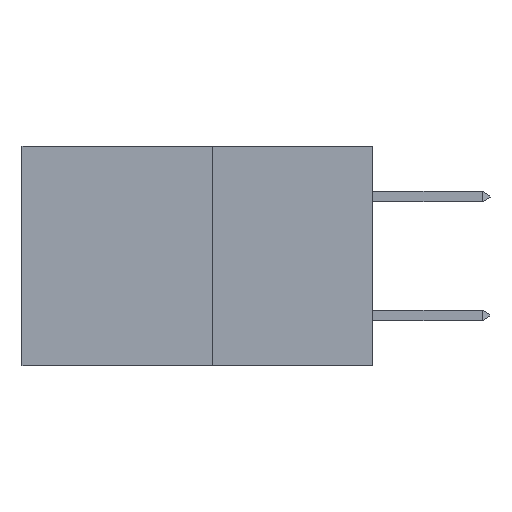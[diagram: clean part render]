
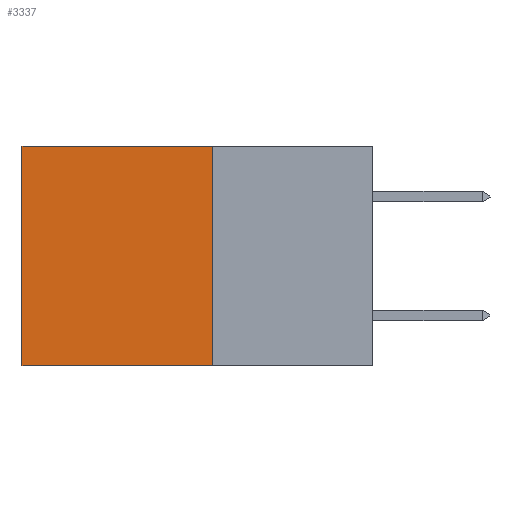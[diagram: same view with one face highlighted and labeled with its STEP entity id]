
A CAD part, left-side view. The second image highlights one B-rep face of the part: STEP entity #3337.
In plain terms, the highlighted planar face has unit normal (-1, 0, 0).
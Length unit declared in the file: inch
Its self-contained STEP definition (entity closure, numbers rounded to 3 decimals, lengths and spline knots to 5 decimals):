
#795 = DIRECTION ( 'NONE',  ( 0., 1., 0. ) ) ;
#839 = CARTESIAN_POINT ( 'NONE',  ( 0.277, 0.27, -0.37 ) ) ;
#1042 = VERTEX_POINT ( 'NONE', #9875 ) ;
#1061 = ORIENTED_EDGE ( 'NONE', *, *, #6107, .T. ) ;
#1336 = EDGE_CURVE ( 'NONE', #9723, #1696, #6829, .T. ) ;
#1437 = ORIENTED_EDGE ( 'NONE', *, *, #1336, .F. ) ;
#1644 = DIRECTION ( 'NONE',  ( 0., 1., 0. ) ) ;
#1651 = EDGE_CURVE ( 'NONE', #9723, #1042, #3816, .T. ) ;
#1696 = VERTEX_POINT ( 'NONE', #1767 ) ;
#1767 = CARTESIAN_POINT ( 'NONE',  ( 0.277, 0.27, -0.37 ) ) ;
#2977 = VECTOR ( 'NONE', #11805, 39.37008 ) ;
#3291 = CARTESIAN_POINT ( 'NONE',  ( 0.277, 0.59, -0.37 ) ) ;
#3337 = ADVANCED_FACE ( 'NONE', ( #3777 ), #9897, .F. ) ;
#3438 = EDGE_CURVE ( 'NONE', #1696, #5082, #12374, .T. ) ;
#3777 = FACE_OUTER_BOUND ( 'NONE', #3894, .T. ) ;
#3816 = LINE ( 'NONE', #8935, #8815 ) ;
#3894 = EDGE_LOOP ( 'NONE', ( #1061, #6743, #1437, #8344 ) ) ;
#5082 = VERTEX_POINT ( 'NONE', #3291 ) ;
#5830 = LINE ( 'NONE', #10865, #2977 ) ;
#6107 = EDGE_CURVE ( 'NONE', #1042, #5082, #5830, .T. ) ;
#6743 = ORIENTED_EDGE ( 'NONE', *, *, #3438, .F. ) ;
#6829 = LINE ( 'NONE', #10586, #9134 ) ;
#7911 = CARTESIAN_POINT ( 'NONE',  ( 0.277, 0.27, 0. ) ) ;
#8344 = ORIENTED_EDGE ( 'NONE', *, *, #1651, .T. ) ;
#8815 = VECTOR ( 'NONE', #1644, 39.37008 ) ;
#8935 = CARTESIAN_POINT ( 'NONE',  ( 0.277, 0.27, 0. ) ) ;
#9134 = VECTOR ( 'NONE', #9877, 39.37008 ) ;
#9723 = VERTEX_POINT ( 'NONE', #7911 ) ;
#9742 = DIRECTION ( 'NONE',  ( 0., 0., -1. ) ) ;
#9764 = DIRECTION ( 'NONE',  ( 1., 0., 0. ) ) ;
#9875 = CARTESIAN_POINT ( 'NONE',  ( 0.277, 0.59, 0. ) ) ;
#9877 = DIRECTION ( 'NONE',  ( 0., 0., -1. ) ) ;
#9897 = PLANE ( 'NONE',  #10129 ) ;
#10129 = AXIS2_PLACEMENT_3D ( 'NONE', #10610, #9764, #9742 ) ;
#10586 = CARTESIAN_POINT ( 'NONE',  ( 0.277, 0.27, -0.37 ) ) ;
#10610 = CARTESIAN_POINT ( 'NONE',  ( 0.277, 0.27, -0.37 ) ) ;
#10865 = CARTESIAN_POINT ( 'NONE',  ( 0.277, 0.59, -0.37 ) ) ;
#11805 = DIRECTION ( 'NONE',  ( 0., 0., -1. ) ) ;
#12374 = LINE ( 'NONE', #839, #12670 ) ;
#12670 = VECTOR ( 'NONE', #795, 39.37008 ) ;
